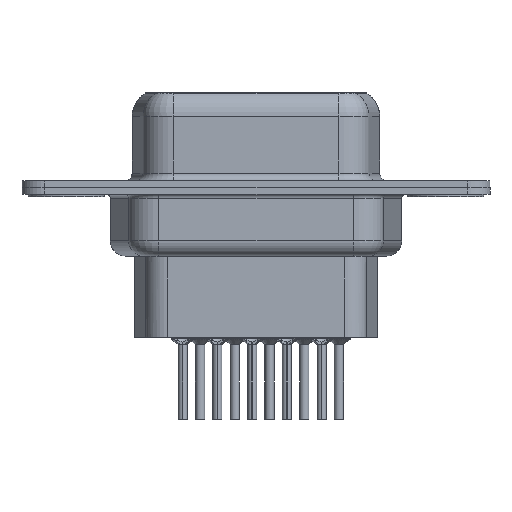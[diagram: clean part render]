
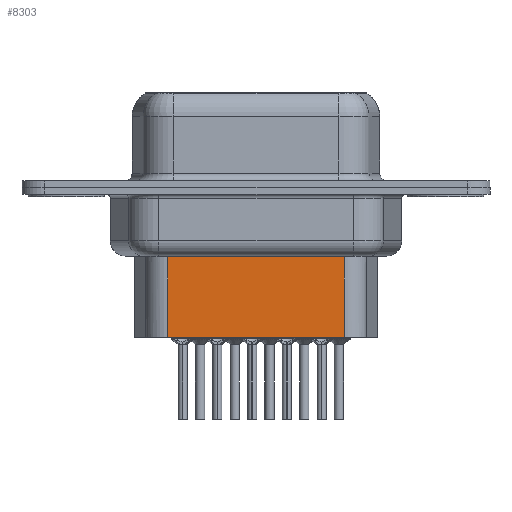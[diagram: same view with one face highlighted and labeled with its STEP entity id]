
A CAD part, front view. The second image highlights one B-rep face of the part: STEP entity #8303.
In plain terms, the highlighted planar face has unit normal (0, -1, 0).
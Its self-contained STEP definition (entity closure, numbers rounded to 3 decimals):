
#996 = FACE_OUTER_BOUND ( 'NONE', #11540, .T. ) ;
#3047 = EDGE_CURVE ( 'NONE', #6416, #25760, #6788, .T. ) ;
#4673 = PLANE ( 'NONE',  #10106 ) ;
#4683 = LINE ( 'NONE', #8101, #10752 ) ;
#5158 = CARTESIAN_POINT ( 'NONE',  ( 6.454, -3.5, -4.097 ) ) ;
#6416 = VERTEX_POINT ( 'NONE', #17661 ) ;
#6717 = CARTESIAN_POINT ( 'NONE',  ( 6.701, -3.5, -3.1 ) ) ;
#6788 = LINE ( 'NONE', #16274, #17084 ) ;
#8101 = CARTESIAN_POINT ( 'NONE',  ( 6.701, -3.5, -9.85 ) ) ;
#8303 = ADVANCED_FACE ( 'NONE', ( #996 ), #4673, .T. ) ;
#8610 = VERTEX_POINT ( 'NONE', #20040 ) ;
#8786 = DIRECTION ( 'NONE',  ( 1., 0., 0. ) ) ;
#10106 = AXIS2_PLACEMENT_3D ( 'NONE', #6717, #21056, #8786 ) ;
#10154 = DIRECTION ( 'NONE',  ( 0., 0., -1. ) ) ;
#10249 = DIRECTION ( 'NONE',  ( -1., 0., 0. ) ) ;
#10752 = VECTOR ( 'NONE', #10249, 1000. ) ;
#11540 = EDGE_LOOP ( 'NONE', ( #19187, #12821, #12443, #12749 ) ) ;
#12443 = ORIENTED_EDGE ( 'NONE', *, *, #26450, .T. ) ;
#12681 = DIRECTION ( 'NONE',  ( 0., 0., -1. ) ) ;
#12749 = ORIENTED_EDGE ( 'NONE', *, *, #20203, .F. ) ;
#12821 = ORIENTED_EDGE ( 'NONE', *, *, #21471, .T. ) ;
#14263 = LINE ( 'NONE', #5158, #20333 ) ;
#14489 = CARTESIAN_POINT ( 'NONE',  ( 6.701, -3.5, -4.097 ) ) ;
#14909 = VECTOR ( 'NONE', #12681, 1000. ) ;
#16274 = CARTESIAN_POINT ( 'NONE',  ( 18.289, -3.5, -3.1 ) ) ;
#17084 = VECTOR ( 'NONE', #10154, 1000. ) ;
#17661 = CARTESIAN_POINT ( 'NONE',  ( 18.289, -3.5, -4.097 ) ) ;
#18178 = CARTESIAN_POINT ( 'NONE',  ( 18.289, -3.5, -9.85 ) ) ;
#18781 = CARTESIAN_POINT ( 'NONE',  ( 6.701, -3.5, -3.1 ) ) ;
#19187 = ORIENTED_EDGE ( 'NONE', *, *, #3047, .F. ) ;
#19500 = DIRECTION ( 'NONE',  ( -1., 0., 0. ) ) ;
#20040 = CARTESIAN_POINT ( 'NONE',  ( 6.701, -3.5, -9.85 ) ) ;
#20203 = EDGE_CURVE ( 'NONE', #25760, #8610, #4683, .T. ) ;
#20333 = VECTOR ( 'NONE', #19500, 1000. ) ;
#20337 = LINE ( 'NONE', #18781, #14909 ) ;
#21056 = DIRECTION ( 'NONE',  ( 0., -1., 0. ) ) ;
#21471 = EDGE_CURVE ( 'NONE', #6416, #24905, #14263, .T. ) ;
#24905 = VERTEX_POINT ( 'NONE', #14489 ) ;
#25760 = VERTEX_POINT ( 'NONE', #18178 ) ;
#26450 = EDGE_CURVE ( 'NONE', #24905, #8610, #20337, .T. ) ;
